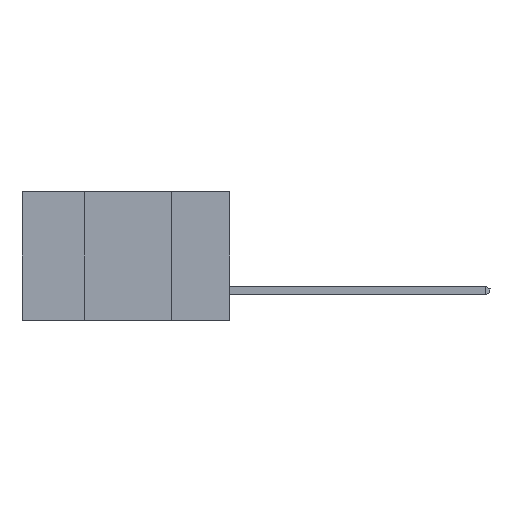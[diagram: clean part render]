
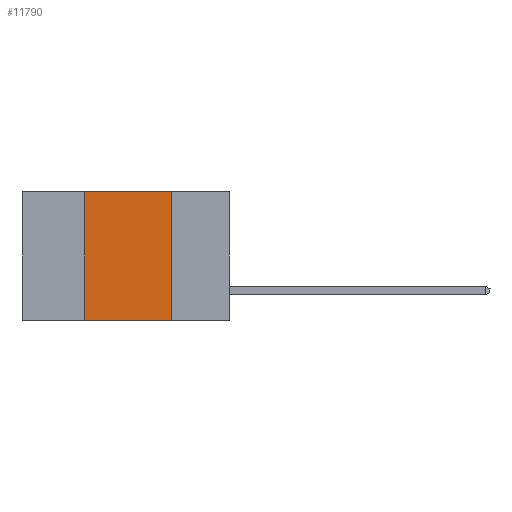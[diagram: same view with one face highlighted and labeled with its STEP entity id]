
A CAD part, left-side view. The second image highlights one B-rep face of the part: STEP entity #11790.
In plain terms, the highlighted planar face has unit normal (-1, 0, 0).
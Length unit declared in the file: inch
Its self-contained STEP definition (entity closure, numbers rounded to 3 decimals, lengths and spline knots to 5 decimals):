
#137 = EDGE_CURVE ( 'NONE', #14364, #18387, #3438, .T. ) ;
#591 = CARTESIAN_POINT ( 'NONE',  ( 0., 0.17, -0.37 ) ) ;
#1284 = ORIENTED_EDGE ( 'NONE', *, *, #3423, .F. ) ;
#1652 = DIRECTION ( 'NONE',  ( 1., 0., 0. ) ) ;
#2285 = ORIENTED_EDGE ( 'NONE', *, *, #137, .F. ) ;
#2571 = DIRECTION ( 'NONE',  ( 0., 0., -1. ) ) ;
#2614 = DIRECTION ( 'NONE',  ( 0., -1., 0. ) ) ;
#3167 = CARTESIAN_POINT ( 'NONE',  ( 0., 0.42, 0. ) ) ;
#3423 = EDGE_CURVE ( 'NONE', #22056, #14364, #17456, .T. ) ;
#3438 = LINE ( 'NONE', #25577, #23761 ) ;
#3641 = PLANE ( 'NONE',  #19586 ) ;
#4272 = EDGE_CURVE ( 'NONE', #22056, #16813, #8578, .T. ) ;
#5165 = DIRECTION ( 'NONE',  ( 0., -1., 0. ) ) ;
#6685 = LINE ( 'NONE', #591, #9017 ) ;
#8578 = LINE ( 'NONE', #25265, #15585 ) ;
#9017 = VECTOR ( 'NONE', #2571, 39.37008 ) ;
#9230 = FACE_OUTER_BOUND ( 'NONE', #11566, .T. ) ;
#10565 = CARTESIAN_POINT ( 'NONE',  ( 0., 0.42, -0.37 ) ) ;
#10627 = VECTOR ( 'NONE', #13417, 39.37008 ) ;
#11349 = ORIENTED_EDGE ( 'NONE', *, *, #4272, .T. ) ;
#11566 = EDGE_LOOP ( 'NONE', ( #24573, #2285, #1284, #11349 ) ) ;
#11604 = DIRECTION ( 'NONE',  ( 0., 0., -1. ) ) ;
#11790 = ADVANCED_FACE ( 'NONE', ( #9230 ), #3641, .F. ) ;
#13417 = DIRECTION ( 'NONE',  ( 0., 0., 1. ) ) ;
#14364 = VERTEX_POINT ( 'NONE', #3167 ) ;
#15585 = VECTOR ( 'NONE', #2614, 39.37008 ) ;
#16555 = CARTESIAN_POINT ( 'NONE',  ( 0., 0.17, -0.37 ) ) ;
#16813 = VERTEX_POINT ( 'NONE', #16555 ) ;
#17456 = LINE ( 'NONE', #19201, #10627 ) ;
#18387 = VERTEX_POINT ( 'NONE', #18648 ) ;
#18648 = CARTESIAN_POINT ( 'NONE',  ( 0., 0.17, 0. ) ) ;
#19201 = CARTESIAN_POINT ( 'NONE',  ( 0., 0.42, -0.37 ) ) ;
#19586 = AXIS2_PLACEMENT_3D ( 'NONE', #21769, #1652, #11604 ) ;
#21328 = EDGE_CURVE ( 'NONE', #18387, #16813, #6685, .T. ) ;
#21769 = CARTESIAN_POINT ( 'NONE',  ( 0., 0.6, 0. ) ) ;
#22056 = VERTEX_POINT ( 'NONE', #10565 ) ;
#23761 = VECTOR ( 'NONE', #5165, 39.37008 ) ;
#24573 = ORIENTED_EDGE ( 'NONE', *, *, #21328, .F. ) ;
#25265 = CARTESIAN_POINT ( 'NONE',  ( 0., 0.6, -0.37 ) ) ;
#25577 = CARTESIAN_POINT ( 'NONE',  ( 0., 0.6, 0. ) ) ;
